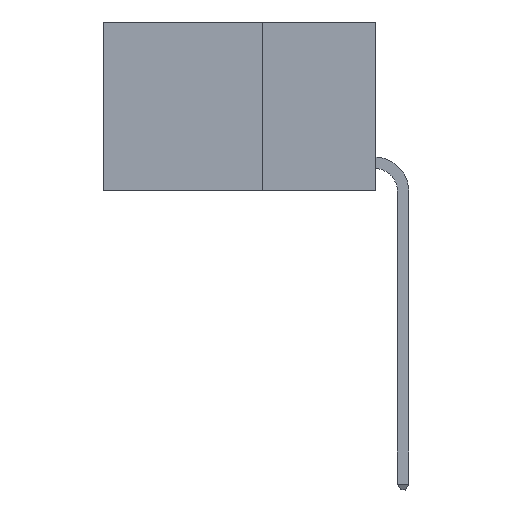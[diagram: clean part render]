
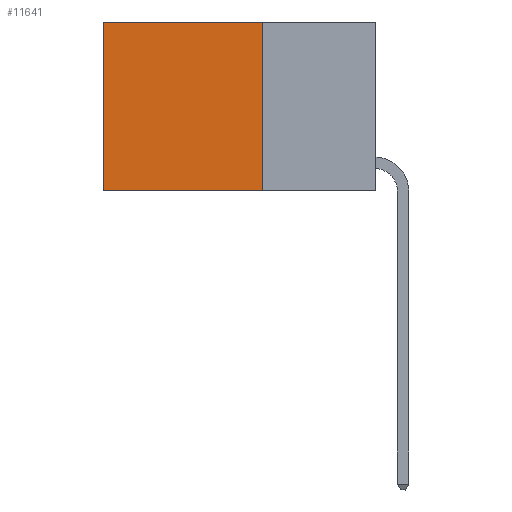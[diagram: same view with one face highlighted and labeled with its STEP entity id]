
A CAD part, left-side view. The second image highlights one B-rep face of the part: STEP entity #11641.
In plain terms, the highlighted planar face has unit normal (-1, 0, 0).
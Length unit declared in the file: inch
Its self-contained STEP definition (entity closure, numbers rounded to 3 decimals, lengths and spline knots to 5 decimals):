
#2292 = EDGE_CURVE ( 'NONE', #13637, #18579, #12655, .T. ) ;
#2615 = LINE ( 'NONE', #3022, #12135 ) ;
#2717 = VECTOR ( 'NONE', #11732, 39.37008 ) ;
#3022 = CARTESIAN_POINT ( 'NONE',  ( 0.2625, 0.25, 0. ) ) ;
#3268 = CARTESIAN_POINT ( 'NONE',  ( 0.2625, 0.25, 0. ) ) ;
#3389 = CARTESIAN_POINT ( 'NONE',  ( 0.2625, 0.25, -0.37 ) ) ;
#5009 = VERTEX_POINT ( 'NONE', #6685 ) ;
#5102 = ORIENTED_EDGE ( 'NONE', *, *, #2292, .F. ) ;
#5827 = EDGE_CURVE ( 'NONE', #12619, #5009, #18609, .T. ) ;
#6685 = CARTESIAN_POINT ( 'NONE',  ( 0.2625, 0.6, -0.37 ) ) ;
#6816 = PLANE ( 'NONE',  #21892 ) ;
#8734 = DIRECTION ( 'NONE',  ( 0., 0., -1. ) ) ;
#9763 = VECTOR ( 'NONE', #16576, 39.37008 ) ;
#11383 = CARTESIAN_POINT ( 'NONE',  ( 0.2625, 0.6, 0. ) ) ;
#11641 = ADVANCED_FACE ( 'NONE', ( #21592 ), #6816, .F. ) ;
#11666 = CARTESIAN_POINT ( 'NONE',  ( 0.2625, 0.25, -0.37 ) ) ;
#11732 = DIRECTION ( 'NONE',  ( 0., 1., 0. ) ) ;
#12135 = VECTOR ( 'NONE', #15487, 39.37008 ) ;
#12187 = EDGE_LOOP ( 'NONE', ( #18154, #14043, #5102, #15147 ) ) ;
#12262 = CARTESIAN_POINT ( 'NONE',  ( 0.2625, 0.25, 0. ) ) ;
#12619 = VERTEX_POINT ( 'NONE', #11383 ) ;
#12655 = LINE ( 'NONE', #20097, #13207 ) ;
#12777 = EDGE_CURVE ( 'NONE', #18579, #5009, #12782, .T. ) ;
#12782 = LINE ( 'NONE', #11666, #2717 ) ;
#13207 = VECTOR ( 'NONE', #14794, 39.37008 ) ;
#13637 = VERTEX_POINT ( 'NONE', #3268 ) ;
#14043 = ORIENTED_EDGE ( 'NONE', *, *, #12777, .F. ) ;
#14794 = DIRECTION ( 'NONE',  ( 0., 0., -1. ) ) ;
#14801 = CARTESIAN_POINT ( 'NONE',  ( 0.2625, 0.6, 0. ) ) ;
#15147 = ORIENTED_EDGE ( 'NONE', *, *, #20912, .T. ) ;
#15487 = DIRECTION ( 'NONE',  ( 0., 1., 0. ) ) ;
#16576 = DIRECTION ( 'NONE',  ( 0., 0., -1. ) ) ;
#18154 = ORIENTED_EDGE ( 'NONE', *, *, #5827, .T. ) ;
#18579 = VERTEX_POINT ( 'NONE', #3389 ) ;
#18609 = LINE ( 'NONE', #14801, #9763 ) ;
#19357 = DIRECTION ( 'NONE',  ( 1., 0., 0. ) ) ;
#20097 = CARTESIAN_POINT ( 'NONE',  ( 0.2625, 0.25, 0. ) ) ;
#20912 = EDGE_CURVE ( 'NONE', #13637, #12619, #2615, .T. ) ;
#21592 = FACE_OUTER_BOUND ( 'NONE', #12187, .T. ) ;
#21892 = AXIS2_PLACEMENT_3D ( 'NONE', #12262, #19357, #8734 ) ;
